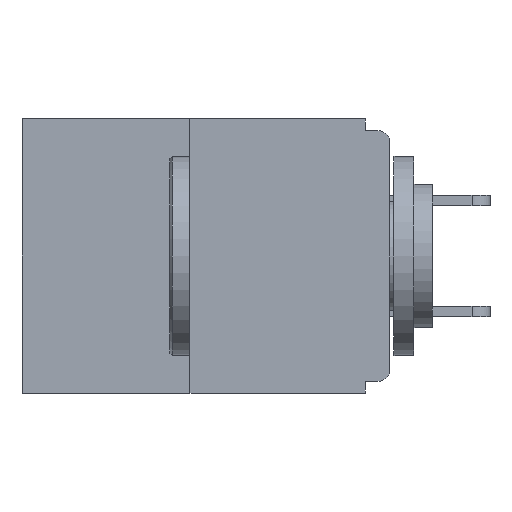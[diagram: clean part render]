
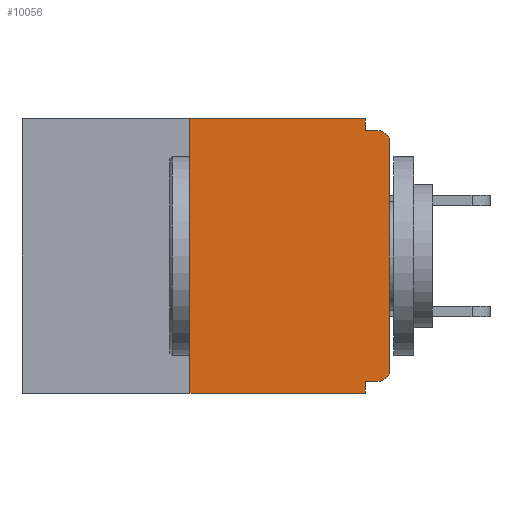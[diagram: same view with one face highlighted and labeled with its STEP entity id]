
A CAD part, left-side view. The second image highlights one B-rep face of the part: STEP entity #10056.
In plain terms, the highlighted planar face has unit normal (-1, 0, 0).
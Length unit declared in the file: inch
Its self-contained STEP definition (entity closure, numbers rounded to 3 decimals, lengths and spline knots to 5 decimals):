
#644 = LINE ( 'NONE', #20298, #3494 ) ;
#786 = VECTOR ( 'NONE', #3782, 39.37008 ) ;
#1155 = VECTOR ( 'NONE', #8791, 39.37008 ) ;
#1364 = CARTESIAN_POINT ( 'NONE',  ( 0., 0.25, 0. ) ) ;
#1902 = EDGE_CURVE ( 'NONE', #22506, #20297, #14707, .T. ) ;
#2053 = EDGE_CURVE ( 'NONE', #14286, #26089, #22339, .T. ) ;
#2654 = CARTESIAN_POINT ( 'NONE',  ( 0., 0.031, -0.343 ) ) ;
#2777 = CARTESIAN_POINT ( 'NONE',  ( 0., 0., -0.015 ) ) ;
#3354 = EDGE_CURVE ( 'NONE', #3799, #16517, #12411, .T. ) ;
#3494 = VECTOR ( 'NONE', #17914, 39.37008 ) ;
#3504 = DIRECTION ( 'NONE',  ( 1., 0., 0. ) ) ;
#3507 = ORIENTED_EDGE ( 'NONE', *, *, #19577, .F. ) ;
#3628 = DIRECTION ( 'NONE',  ( -1., 0., 0. ) ) ;
#3665 = CARTESIAN_POINT ( 'NONE',  ( 0., 0.015, -0.313 ) ) ;
#3782 = DIRECTION ( 'NONE',  ( 0., 0., -1. ) ) ;
#3799 = VERTEX_POINT ( 'NONE', #9228 ) ;
#4280 = CARTESIAN_POINT ( 'NONE',  ( 0., 0.031, -0.328 ) ) ;
#4369 = VECTOR ( 'NONE', #5482, 39.37008 ) ;
#4564 = ORIENTED_EDGE ( 'NONE', *, *, #23280, .F. ) ;
#5362 = PLANE ( 'NONE',  #5568 ) ;
#5471 = CARTESIAN_POINT ( 'NONE',  ( 0., 0., -0.313 ) ) ;
#5482 = DIRECTION ( 'NONE',  ( 0., -1., 0. ) ) ;
#5568 = AXIS2_PLACEMENT_3D ( 'NONE', #15580, #3504, #11616 ) ;
#5861 = DIRECTION ( 'NONE',  ( 0., 0., -1. ) ) ;
#6925 = AXIS2_PLACEMENT_3D ( 'NONE', #21941, #3628, #23899 ) ;
#7690 = CARTESIAN_POINT ( 'NONE',  ( 0., 0., -0.03 ) ) ;
#8208 = EDGE_CURVE ( 'NONE', #14286, #24466, #23598, .T. ) ;
#8240 = EDGE_LOOP ( 'NONE', ( #4564, #9643, #24813, #11340, #9945, #9423, #14855, #16379, #3507, #22167 ) ) ;
#8791 = DIRECTION ( 'NONE',  ( 0., -1., 0. ) ) ;
#8959 = CARTESIAN_POINT ( 'NONE',  ( 0., 0.46, -0.343 ) ) ;
#9007 = DIRECTION ( 'NONE',  ( 0., 0., 1. ) ) ;
#9118 = CARTESIAN_POINT ( 'NONE',  ( 0., 0., -0.328 ) ) ;
#9173 = CARTESIAN_POINT ( 'NONE',  ( 0., 0.25, -0.343 ) ) ;
#9228 = CARTESIAN_POINT ( 'NONE',  ( 0., 0.015, -0.328 ) ) ;
#9423 = ORIENTED_EDGE ( 'NONE', *, *, #20215, .T. ) ;
#9643 = ORIENTED_EDGE ( 'NONE', *, *, #2053, .F. ) ;
#9799 = VERTEX_POINT ( 'NONE', #5471 ) ;
#9945 = ORIENTED_EDGE ( 'NONE', *, *, #3354, .F. ) ;
#10056 = ADVANCED_FACE ( 'NONE', ( #24537 ), #5362, .F. ) ;
#10702 = CARTESIAN_POINT ( 'NONE',  ( 0., 0., 0. ) ) ;
#11250 = AXIS2_PLACEMENT_3D ( 'NONE', #3665, #24202, #5861 ) ;
#11265 = VERTEX_POINT ( 'NONE', #7690 ) ;
#11275 = CIRCLE ( 'NONE', #6925, 0.015 ) ;
#11280 = CARTESIAN_POINT ( 'NONE',  ( 0., 0.25, 0. ) ) ;
#11340 = ORIENTED_EDGE ( 'NONE', *, *, #17789, .F. ) ;
#11616 = DIRECTION ( 'NONE',  ( 0., 0., -1. ) ) ;
#12411 = LINE ( 'NONE', #9118, #21318 ) ;
#12655 = CARTESIAN_POINT ( 'NONE',  ( 0., 0.015, -0.015 ) ) ;
#12850 = VECTOR ( 'NONE', #18920, 39.37008 ) ;
#13065 = DIRECTION ( 'NONE',  ( 0., 1., 0. ) ) ;
#14286 = VERTEX_POINT ( 'NONE', #9173 ) ;
#14707 = LINE ( 'NONE', #15884, #786 ) ;
#14845 = DIRECTION ( 'NONE',  ( 0., -1., 0. ) ) ;
#14855 = ORIENTED_EDGE ( 'NONE', *, *, #19907, .T. ) ;
#15410 = CARTESIAN_POINT ( 'NONE',  ( 0., 0.031, 0. ) ) ;
#15580 = CARTESIAN_POINT ( 'NONE',  ( 0., 0.46, 0. ) ) ;
#15884 = CARTESIAN_POINT ( 'NONE',  ( 0., 0.031, 0. ) ) ;
#16379 = ORIENTED_EDGE ( 'NONE', *, *, #24245, .T. ) ;
#16517 = VERTEX_POINT ( 'NONE', #4280 ) ;
#17312 = LINE ( 'NONE', #2777, #1155 ) ;
#17517 = CARTESIAN_POINT ( 'NONE',  ( 0., 0.46, 0. ) ) ;
#17789 = EDGE_CURVE ( 'NONE', #16517, #24466, #644, .T. ) ;
#17914 = DIRECTION ( 'NONE',  ( 0., 0., -1. ) ) ;
#18920 = DIRECTION ( 'NONE',  ( 0., 0., 1. ) ) ;
#19571 = VERTEX_POINT ( 'NONE', #12655 ) ;
#19577 = EDGE_CURVE ( 'NONE', #20297, #19571, #17312, .T. ) ;
#19907 = EDGE_CURVE ( 'NONE', #9799, #11265, #21724, .T. ) ;
#20215 = EDGE_CURVE ( 'NONE', #3799, #9799, #24900, .T. ) ;
#20297 = VERTEX_POINT ( 'NONE', #20570 ) ;
#20298 = CARTESIAN_POINT ( 'NONE',  ( 0., 0.031, -0.343 ) ) ;
#20570 = CARTESIAN_POINT ( 'NONE',  ( 0., 0.031, -0.015 ) ) ;
#21318 = VECTOR ( 'NONE', #13065, 39.37008 ) ;
#21724 = LINE ( 'NONE', #10702, #12850 ) ;
#21941 = CARTESIAN_POINT ( 'NONE',  ( 0., 0.015, -0.03 ) ) ;
#22167 = ORIENTED_EDGE ( 'NONE', *, *, #1902, .F. ) ;
#22339 = LINE ( 'NONE', #11280, #23596 ) ;
#22506 = VERTEX_POINT ( 'NONE', #15410 ) ;
#23280 = EDGE_CURVE ( 'NONE', #26089, #22506, #25895, .T. ) ;
#23596 = VECTOR ( 'NONE', #9007, 39.37008 ) ;
#23598 = LINE ( 'NONE', #8959, #23639 ) ;
#23639 = VECTOR ( 'NONE', #14845, 39.37008 ) ;
#23899 = DIRECTION ( 'NONE',  ( 0., 0., -1. ) ) ;
#24202 = DIRECTION ( 'NONE',  ( -1., 0., 0. ) ) ;
#24245 = EDGE_CURVE ( 'NONE', #11265, #19571, #11275, .T. ) ;
#24466 = VERTEX_POINT ( 'NONE', #2654 ) ;
#24537 = FACE_OUTER_BOUND ( 'NONE', #8240, .T. ) ;
#24813 = ORIENTED_EDGE ( 'NONE', *, *, #8208, .T. ) ;
#24900 = CIRCLE ( 'NONE', #11250, 0.015 ) ;
#25895 = LINE ( 'NONE', #17517, #4369 ) ;
#26089 = VERTEX_POINT ( 'NONE', #1364 ) ;
